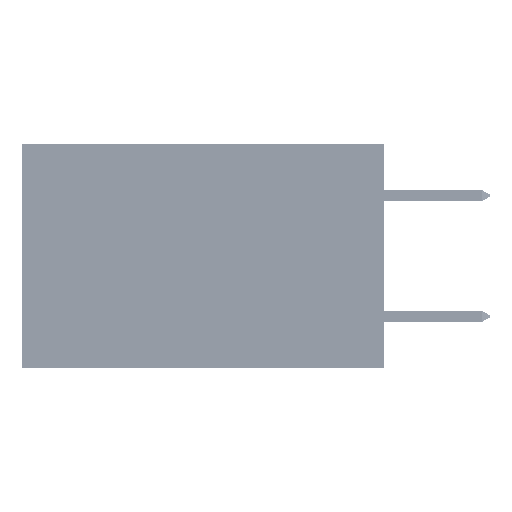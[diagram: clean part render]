
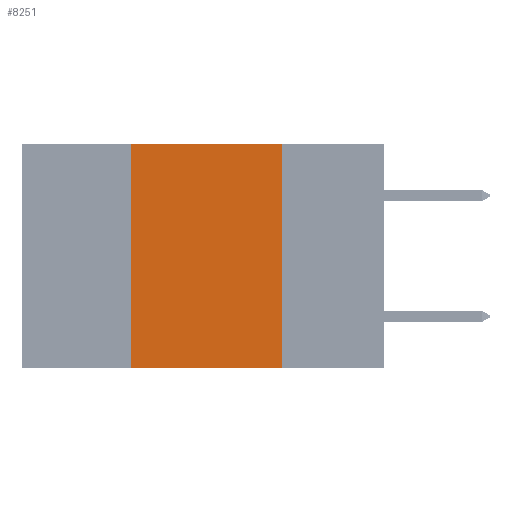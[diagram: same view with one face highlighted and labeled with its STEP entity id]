
A CAD part, left-side view. The second image highlights one B-rep face of the part: STEP entity #8251.
In plain terms, the highlighted planar face has unit normal (-1, 0, 0).
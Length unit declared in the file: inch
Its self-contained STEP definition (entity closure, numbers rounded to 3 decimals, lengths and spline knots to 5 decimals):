
#576 = LINE ( 'NONE', #33673, #7511 ) ;
#604 = CARTESIAN_POINT ( 'NONE',  ( 0., 0.42, -0.37 ) ) ;
#831 = CARTESIAN_POINT ( 'NONE',  ( 0., 0.17, 0. ) ) ;
#2650 = EDGE_LOOP ( 'NONE', ( #4023, #7396, #29888, #28659 ) ) ;
#4023 = ORIENTED_EDGE ( 'NONE', *, *, #34424, .F. ) ;
#4686 = FACE_OUTER_BOUND ( 'NONE', #2650, .T. ) ;
#5230 = CARTESIAN_POINT ( 'NONE',  ( 0., 0.42, 0. ) ) ;
#5702 = LINE ( 'NONE', #22939, #22038 ) ;
#6259 = VERTEX_POINT ( 'NONE', #5230 ) ;
#6603 = CARTESIAN_POINT ( 'NONE',  ( 0., 0.17, 0. ) ) ;
#7396 = ORIENTED_EDGE ( 'NONE', *, *, #14798, .F. ) ;
#7511 = VECTOR ( 'NONE', #22014, 39.37008 ) ;
#8251 = ADVANCED_FACE ( 'NONE', ( #4686 ), #34446, .F. ) ;
#14798 = EDGE_CURVE ( 'NONE', #6259, #34582, #27339, .T. ) ;
#17966 = VERTEX_POINT ( 'NONE', #46073 ) ;
#19093 = CARTESIAN_POINT ( 'NONE',  ( 0., 0.6, 0. ) ) ;
#19142 = VECTOR ( 'NONE', #26448, 39.37008 ) ;
#19763 = LINE ( 'NONE', #831, #51847 ) ;
#21638 = EDGE_CURVE ( 'NONE', #51281, #6259, #5702, .T. ) ;
#22012 = CARTESIAN_POINT ( 'NONE',  ( 0., 0.6, 0. ) ) ;
#22014 = DIRECTION ( 'NONE',  ( 0., -1., 0. ) ) ;
#22038 = VECTOR ( 'NONE', #42886, 39.37008 ) ;
#22939 = CARTESIAN_POINT ( 'NONE',  ( 0., 0.42, 0. ) ) ;
#26448 = DIRECTION ( 'NONE',  ( 0., -1., 0. ) ) ;
#27222 = EDGE_CURVE ( 'NONE', #51281, #17966, #576, .T. ) ;
#27339 = LINE ( 'NONE', #22012, #19142 ) ;
#28659 = ORIENTED_EDGE ( 'NONE', *, *, #27222, .T. ) ;
#29888 = ORIENTED_EDGE ( 'NONE', *, *, #21638, .F. ) ;
#33673 = CARTESIAN_POINT ( 'NONE',  ( 0., 0.6, -0.37 ) ) ;
#34424 = EDGE_CURVE ( 'NONE', #34582, #17966, #19763, .T. ) ;
#34446 = PLANE ( 'NONE',  #37172 ) ;
#34582 = VERTEX_POINT ( 'NONE', #6603 ) ;
#37172 = AXIS2_PLACEMENT_3D ( 'NONE', #19093, #38480, #47258 ) ;
#38480 = DIRECTION ( 'NONE',  ( 1., 0., 0. ) ) ;
#42886 = DIRECTION ( 'NONE',  ( 0., 0., 1. ) ) ;
#45525 = DIRECTION ( 'NONE',  ( 0., 0., -1. ) ) ;
#46073 = CARTESIAN_POINT ( 'NONE',  ( 0., 0.17, -0.37 ) ) ;
#47258 = DIRECTION ( 'NONE',  ( 0., 0., -1. ) ) ;
#51281 = VERTEX_POINT ( 'NONE', #604 ) ;
#51847 = VECTOR ( 'NONE', #45525, 39.37008 ) ;
